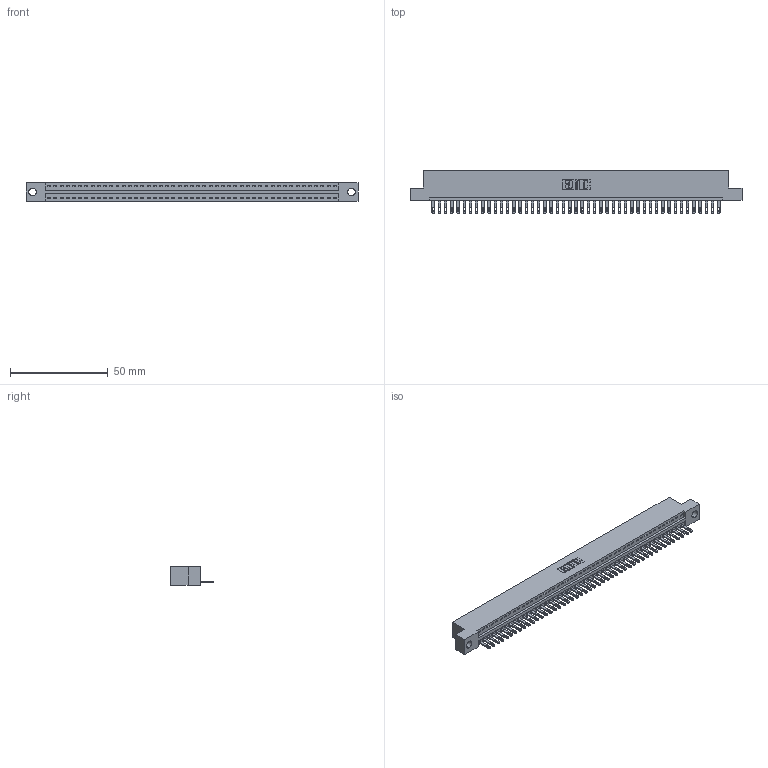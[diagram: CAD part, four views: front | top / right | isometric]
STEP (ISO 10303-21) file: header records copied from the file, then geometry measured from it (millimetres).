
FILE_DESCRIPTION (( 'STEP AP203' ), '1' );
FILE_NAME ('896-047-500-104.STEP', '2021-07-27T22:45:51', ( '' ), ( '' ), 'SwSTEP 2.0', 'SolidWorks 2020', '' );
FILE_SCHEMA (( 'CONFIG_CONTROL_DESIGN' ));
Length unit declared in the file: inch
Products named in the file (3): 345-292-001_345-293-100; 846 Part_Flush Mounting Lugs - 0.156 Dia-TH; 896-047-500-104
Assembly tree (48 placements, depth 2):
  896-047-500-104
    846 Part_Flush Mounting Lugs - 0.156 Dia-TH
    345-292-001_345-293-100  x47
Bounding box: 169.8 x 21.84 x 9.4 mm (x, y, z)
Volume: 16229.2 mm3; surface area: 20252.9 mm2
Topology: 48 solids, 48 shells, 2660 faces, 8225 edges, 5482 vertices
Faces by surface type: plane 1674, cylinder 986
Entity records: 28429 total; most frequent: CARTESIAN_POINT 4877, ORIENTED_EDGE 4858, DIRECTION 4299, EDGE_CURVE 2429, VECTOR 2105, LINE 2105, VERTEX_POINT 1618, AXIS2_PLACEMENT_3D 1097
